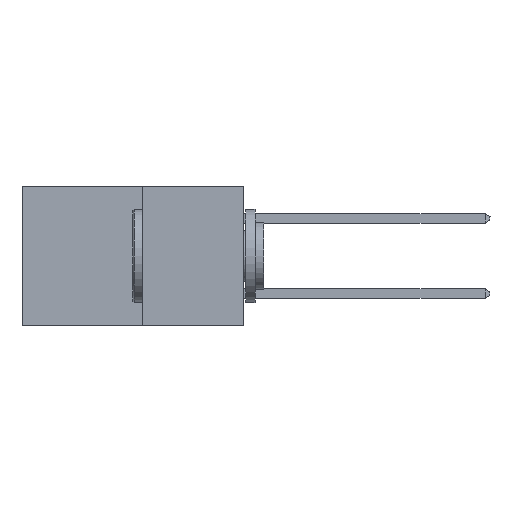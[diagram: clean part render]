
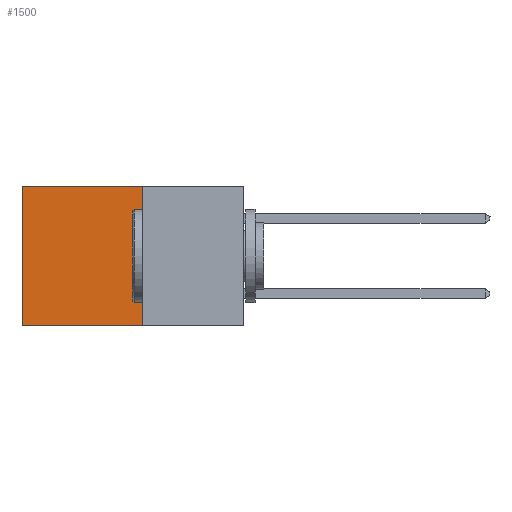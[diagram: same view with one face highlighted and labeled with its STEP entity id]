
A CAD part, left-side view. The second image highlights one B-rep face of the part: STEP entity #1500.
In plain terms, the highlighted planar face has unit normal (-1, 0, 0).
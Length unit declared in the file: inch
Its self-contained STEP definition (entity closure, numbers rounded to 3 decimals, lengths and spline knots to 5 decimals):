
#190 = CARTESIAN_POINT ( 'NONE',  ( 0.277, 0.59, 0. ) ) ;
#923 = VECTOR ( 'NONE', #4304, 39.37008 ) ;
#1092 = FACE_OUTER_BOUND ( 'NONE', #7656, .T. ) ;
#1418 = LINE ( 'NONE', #19750, #17103 ) ;
#1500 = ADVANCED_FACE ( 'NONE', ( #1092 ), #22355, .F. ) ;
#1786 = EDGE_CURVE ( 'NONE', #13011, #21898, #1418, .T. ) ;
#1825 = DIRECTION ( 'NONE',  ( 0., 0., -1. ) ) ;
#4027 = CARTESIAN_POINT ( 'NONE',  ( 0.277, 0.59, -0.37 ) ) ;
#4304 = DIRECTION ( 'NONE',  ( 0., 1., 0. ) ) ;
#4345 = EDGE_CURVE ( 'NONE', #21898, #24680, #6022, .T. ) ;
#4812 = CARTESIAN_POINT ( 'NONE',  ( 0.277, 0.27, -0.37 ) ) ;
#4913 = CARTESIAN_POINT ( 'NONE',  ( 0.277, 0.27, -0.37 ) ) ;
#6022 = LINE ( 'NONE', #4812, #923 ) ;
#7576 = DIRECTION ( 'NONE',  ( 0., 1., 0. ) ) ;
#7656 = EDGE_LOOP ( 'NONE', ( #10580, #10733, #10971, #10975 ) ) ;
#9799 = DIRECTION ( 'NONE',  ( 0., 0., -1. ) ) ;
#10580 = ORIENTED_EDGE ( 'NONE', *, *, #14759, .T. ) ;
#10733 = ORIENTED_EDGE ( 'NONE', *, *, #4345, .F. ) ;
#10764 = CARTESIAN_POINT ( 'NONE',  ( 0.277, 0.27, 0. ) ) ;
#10971 = ORIENTED_EDGE ( 'NONE', *, *, #1786, .F. ) ;
#10975 = ORIENTED_EDGE ( 'NONE', *, *, #18509, .T. ) ;
#13011 = VERTEX_POINT ( 'NONE', #10764 ) ;
#13885 = CARTESIAN_POINT ( 'NONE',  ( 0.277, 0.27, -0.37 ) ) ;
#14759 = EDGE_CURVE ( 'NONE', #26231, #24680, #24518, .T. ) ;
#15564 = DIRECTION ( 'NONE',  ( 1., 0., 0. ) ) ;
#17103 = VECTOR ( 'NONE', #17826, 39.37008 ) ;
#17826 = DIRECTION ( 'NONE',  ( 0., 0., -1. ) ) ;
#18125 = CARTESIAN_POINT ( 'NONE',  ( 0.277, 0.27, 0. ) ) ;
#18509 = EDGE_CURVE ( 'NONE', #13011, #26231, #19624, .T. ) ;
#18855 = VECTOR ( 'NONE', #1825, 39.37008 ) ;
#19054 = CARTESIAN_POINT ( 'NONE',  ( 0.277, 0.59, -0.37 ) ) ;
#19624 = LINE ( 'NONE', #18125, #24631 ) ;
#19750 = CARTESIAN_POINT ( 'NONE',  ( 0.277, 0.27, -0.37 ) ) ;
#21898 = VERTEX_POINT ( 'NONE', #4913 ) ;
#22145 = AXIS2_PLACEMENT_3D ( 'NONE', #13885, #15564, #9799 ) ;
#22355 = PLANE ( 'NONE',  #22145 ) ;
#24518 = LINE ( 'NONE', #4027, #18855 ) ;
#24631 = VECTOR ( 'NONE', #7576, 39.37008 ) ;
#24680 = VERTEX_POINT ( 'NONE', #19054 ) ;
#26231 = VERTEX_POINT ( 'NONE', #190 ) ;
